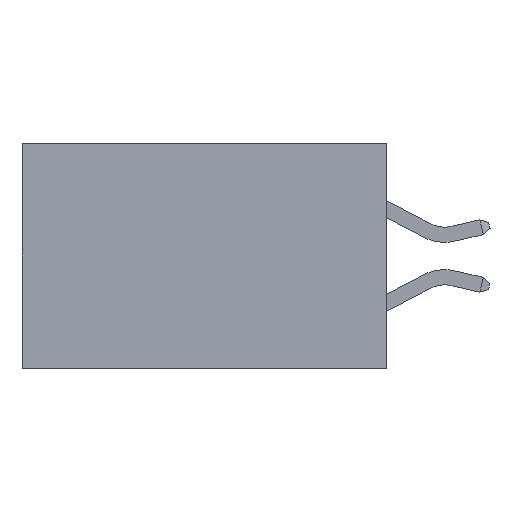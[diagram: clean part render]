
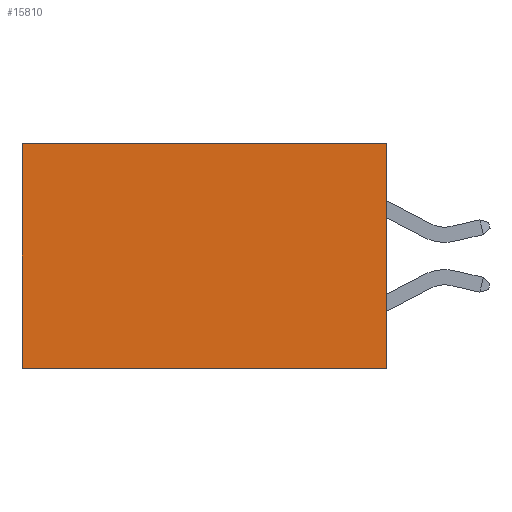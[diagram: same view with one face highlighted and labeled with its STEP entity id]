
A CAD part, left-side view. The second image highlights one B-rep face of the part: STEP entity #15810.
In plain terms, the highlighted planar face has unit normal (-1, 0, 0).
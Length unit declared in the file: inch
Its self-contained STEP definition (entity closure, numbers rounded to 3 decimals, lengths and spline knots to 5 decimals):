
#69 = VERTEX_POINT ( 'NONE', #19444 ) ;
#151 = ORIENTED_EDGE ( 'NONE', *, *, #20360, .F. ) ;
#683 = PLANE ( 'NONE',  #20082 ) ;
#751 = DIRECTION ( 'NONE',  ( 0., 1., 0. ) ) ;
#2417 = DIRECTION ( 'NONE',  ( 0., 0., -1. ) ) ;
#2484 = CARTESIAN_POINT ( 'NONE',  ( 0.298, 0., -0.37 ) ) ;
#3269 = VECTOR ( 'NONE', #18551, 39.37008 ) ;
#4677 = EDGE_LOOP ( 'NONE', ( #9669, #4945, #151, #13534 ) ) ;
#4945 = ORIENTED_EDGE ( 'NONE', *, *, #18260, .F. ) ;
#5567 = CARTESIAN_POINT ( 'NONE',  ( 0.298, 0., 0. ) ) ;
#7526 = DIRECTION ( 'NONE',  ( 0., 0., -1. ) ) ;
#8499 = LINE ( 'NONE', #17742, #10297 ) ;
#8603 = LINE ( 'NONE', #2484, #16654 ) ;
#9669 = ORIENTED_EDGE ( 'NONE', *, *, #13349, .T. ) ;
#10104 = CARTESIAN_POINT ( 'NONE',  ( 0.298, 0., 0. ) ) ;
#10297 = VECTOR ( 'NONE', #19292, 39.37008 ) ;
#10738 = CARTESIAN_POINT ( 'NONE',  ( 0.298, 0., 0. ) ) ;
#11216 = EDGE_CURVE ( 'NONE', #14217, #14957, #16157, .T. ) ;
#12138 = DIRECTION ( 'NONE',  ( 1., 0., 0. ) ) ;
#13305 = VECTOR ( 'NONE', #7526, 39.37008 ) ;
#13349 = EDGE_CURVE ( 'NONE', #14957, #69, #8499, .T. ) ;
#13534 = ORIENTED_EDGE ( 'NONE', *, *, #11216, .T. ) ;
#13825 = LINE ( 'NONE', #10738, #13305 ) ;
#14217 = VERTEX_POINT ( 'NONE', #10104 ) ;
#14957 = VERTEX_POINT ( 'NONE', #16931 ) ;
#15810 = ADVANCED_FACE ( 'NONE', ( #18199 ), #683, .F. ) ;
#16157 = LINE ( 'NONE', #16997, #3269 ) ;
#16374 = VERTEX_POINT ( 'NONE', #19795 ) ;
#16654 = VECTOR ( 'NONE', #751, 39.37008 ) ;
#16931 = CARTESIAN_POINT ( 'NONE',  ( 0.298, 0.6, 0. ) ) ;
#16997 = CARTESIAN_POINT ( 'NONE',  ( 0.298, 0., 0. ) ) ;
#17742 = CARTESIAN_POINT ( 'NONE',  ( 0.298, 0.6, 0. ) ) ;
#18199 = FACE_OUTER_BOUND ( 'NONE', #4677, .T. ) ;
#18260 = EDGE_CURVE ( 'NONE', #16374, #69, #8603, .T. ) ;
#18551 = DIRECTION ( 'NONE',  ( 0., 1., 0. ) ) ;
#19292 = DIRECTION ( 'NONE',  ( 0., 0., -1. ) ) ;
#19444 = CARTESIAN_POINT ( 'NONE',  ( 0.298, 0.6, -0.37 ) ) ;
#19795 = CARTESIAN_POINT ( 'NONE',  ( 0.298, 0., -0.37 ) ) ;
#20082 = AXIS2_PLACEMENT_3D ( 'NONE', #5567, #12138, #2417 ) ;
#20360 = EDGE_CURVE ( 'NONE', #14217, #16374, #13825, .T. ) ;
